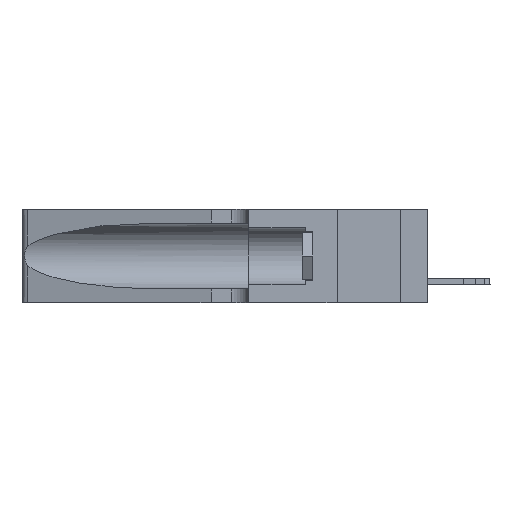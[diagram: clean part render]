
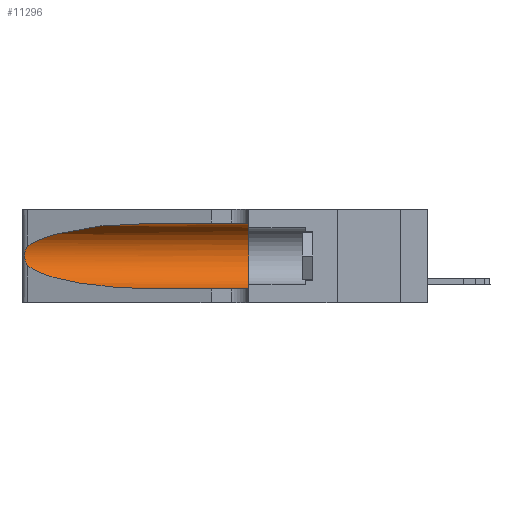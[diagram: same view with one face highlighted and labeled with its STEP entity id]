
A CAD part, left-side view. The second image highlights one B-rep face of the part: STEP entity #11296.
In plain terms, the highlighted cylindrical face has radius 3.308 mm (diameter 6.617 mm), a partial arc.
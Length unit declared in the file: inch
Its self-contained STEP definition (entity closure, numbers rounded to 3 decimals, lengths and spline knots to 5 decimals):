
#935 = CARTESIAN_POINT ( 'NONE',  ( 0.25787, 1.23484, 0.2124 ) ) ;
#1136 = ORIENTED_EDGE ( 'NONE', *, *, #11160, .T. ) ;
#1160 = CARTESIAN_POINT ( 'NONE',  ( 0.25487, 1.22718, 0.14631 ) ) ;
#1245 = VECTOR ( 'NONE', #18800, 39.37008 ) ;
#2476 = CARTESIAN_POINT ( 'NONE',  ( 0.18966, 0.96281, 0.31525 ) ) ;
#2485 = CIRCLE ( 'NONE', #19370, 0.13025 ) ;
#2750 = VERTEX_POINT ( 'NONE', #7155 ) ;
#3383 = CARTESIAN_POINT ( 'NONE',  ( 0.25639, 1.23186, 0.15144 ) ) ;
#3435 = B_SPLINE_CURVE_WITH_KNOTS ( 'NONE', 3,
 ( #26934, #24840, #19873, #935, #5444, #22063, #29535, #5759, #24629, #10415, #15229, #3383, #3483, #20076 ),
 .UNSPECIFIED., .F., .F.,
 ( 4, 2, 2, 2, 2, 2, 4 ),
 ( 0., 0.00027, 0.00053, 0.00107, 0.0016, 0.00187, 0.00214 ),
 .UNSPECIFIED. ) ;
#3483 = CARTESIAN_POINT ( 'NONE',  ( 0.25555, 1.22993, 0.14849 ) ) ;
#3487 = CARTESIAN_POINT ( 'NONE',  ( 0.2373, 1.15595, 0.08982 ) ) ;
#3792 = EDGE_CURVE ( 'NONE', #9569, #2750, #24919, .T. ) ;
#4123 = DIRECTION ( 'NONE',  ( 0., 0., 1. ) ) ;
#4322 = CARTESIAN_POINT ( 'NONE',  ( 0.18966, 0.96281, 0.05475 ) ) ;
#5121 =( BOUNDED_CURVE ( )  B_SPLINE_CURVE ( 3, ( #17701, #3487, #4322, #23492 ),
 .UNSPECIFIED., .F., .T. ) 
 B_SPLINE_CURVE_WITH_KNOTS ( ( 4, 4 ),
 ( 3.44316, 4.71239 ),
 .UNSPECIFIED. ) 
 CURVE ( )  GEOMETRIC_REPRESENTATION_ITEM ( )  RATIONAL_B_SPLINE_CURVE ( ( 1., 0.87, 0.87, 1. ) ) 
 REPRESENTATION_ITEM ( '' )  );
#5444 = CARTESIAN_POINT ( 'NONE',  ( 0.25854, 1.2359, 0.20912 ) ) ;
#5759 = CARTESIAN_POINT ( 'NONE',  ( 0.26075, 1.23896, 0.178 ) ) ;
#6034 = DIRECTION ( 'NONE',  ( 0., 0., -1. ) ) ;
#6055 = EDGE_CURVE ( 'NONE', #29790, #15580, #2485, .T. ) ;
#6140 = ORIENTED_EDGE ( 'NONE', *, *, #18362, .F. ) ;
#7155 = CARTESIAN_POINT ( 'NONE',  ( 0.25487, 1.22718, 0.22369 ) ) ;
#7856 = CYLINDRICAL_SURFACE ( 'NONE', #13748, 0.13025 ) ;
#9201 = DIRECTION ( 'NONE',  ( 0., 1., 0. ) ) ;
#9569 = VERTEX_POINT ( 'NONE', #29063 ) ;
#10415 = CARTESIAN_POINT ( 'NONE',  ( 0.25856, 1.23593, 0.16098 ) ) ;
#11160 = EDGE_CURVE ( 'NONE', #20921, #15580, #15711, .T. ) ;
#11296 = ADVANCED_FACE ( 'NONE', ( #20855 ), #7856, .F. ) ;
#11431 = DIRECTION ( 'NONE',  ( 0., -1., 0. ) ) ;
#11996 = VERTEX_POINT ( 'NONE', #1160 ) ;
#12589 = ORIENTED_EDGE ( 'NONE', *, *, #22698, .T. ) ;
#12838 = EDGE_CURVE ( 'NONE', #11996, #20921, #5121, .T. ) ;
#13206 = CARTESIAN_POINT ( 'NONE',  ( 0.1305, 1.61858, 0.185 ) ) ;
#13689 = CARTESIAN_POINT ( 'NONE',  ( 0.1305, 0.35, 0.185 ) ) ;
#13748 = AXIS2_PLACEMENT_3D ( 'NONE', #13206, #17862, #6034 ) ;
#14402 = CARTESIAN_POINT ( 'NONE',  ( 0.1305, 0.72297, 0.31525 ) ) ;
#14720 = LINE ( 'NONE', #30743, #29181 ) ;
#15229 = CARTESIAN_POINT ( 'NONE',  ( 0.25789, 1.23486, 0.15765 ) ) ;
#15580 = VERTEX_POINT ( 'NONE', #27198 ) ;
#15711 = LINE ( 'NONE', #30462, #1245 ) ;
#16007 = CARTESIAN_POINT ( 'NONE',  ( 0.1305, 0.72297, 0.05475 ) ) ;
#16883 = ORIENTED_EDGE ( 'NONE', *, *, #6055, .F. ) ;
#17701 = CARTESIAN_POINT ( 'NONE',  ( 0.25487, 1.22718, 0.14631 ) ) ;
#17862 = DIRECTION ( 'NONE',  ( 0., -1., 0. ) ) ;
#18316 = EDGE_LOOP ( 'NONE', ( #25067, #12589, #30289, #1136, #16883, #6140 ) ) ;
#18362 = EDGE_CURVE ( 'NONE', #9569, #29790, #14720, .T. ) ;
#18800 = DIRECTION ( 'NONE',  ( 0., -1., 0. ) ) ;
#19036 = CARTESIAN_POINT ( 'NONE',  ( 0.2373, 1.15595, 0.28018 ) ) ;
#19370 = AXIS2_PLACEMENT_3D ( 'NONE', #13689, #9201, #4123 ) ;
#19873 = CARTESIAN_POINT ( 'NONE',  ( 0.25639, 1.23184, 0.21858 ) ) ;
#20076 = CARTESIAN_POINT ( 'NONE',  ( 0.25487, 1.22718, 0.14631 ) ) ;
#20855 = FACE_OUTER_BOUND ( 'NONE', #18316, .T. ) ;
#20921 = VERTEX_POINT ( 'NONE', #16007 ) ;
#22063 = CARTESIAN_POINT ( 'NONE',  ( 0.26018, 1.23835, 0.19895 ) ) ;
#22698 = EDGE_CURVE ( 'NONE', #2750, #11996, #3435, .T. ) ;
#23492 = CARTESIAN_POINT ( 'NONE',  ( 0.1305, 0.72297, 0.05475 ) ) ;
#24629 = CARTESIAN_POINT ( 'NONE',  ( 0.26017, 1.23833, 0.17102 ) ) ;
#24840 = CARTESIAN_POINT ( 'NONE',  ( 0.25555, 1.22994, 0.2215 ) ) ;
#24919 =( BOUNDED_CURVE ( )  B_SPLINE_CURVE ( 3, ( #14402, #2476, #19036, #26406 ),
 .UNSPECIFIED., .F., .T. ) 
 B_SPLINE_CURVE_WITH_KNOTS ( ( 4, 4 ),
 ( 1.5708, 2.84003 ),
 .UNSPECIFIED. ) 
 CURVE ( )  GEOMETRIC_REPRESENTATION_ITEM ( )  RATIONAL_B_SPLINE_CURVE ( ( 1., 0.87, 0.87, 1. ) ) 
 REPRESENTATION_ITEM ( '' )  );
#25067 = ORIENTED_EDGE ( 'NONE', *, *, #3792, .T. ) ;
#26406 = CARTESIAN_POINT ( 'NONE',  ( 0.25487, 1.22718, 0.22369 ) ) ;
#26934 = CARTESIAN_POINT ( 'NONE',  ( 0.25487, 1.22718, 0.22369 ) ) ;
#27198 = CARTESIAN_POINT ( 'NONE',  ( 0.1305, 0.35, 0.05475 ) ) ;
#27576 = CARTESIAN_POINT ( 'NONE',  ( 0.1305, 0.35, 0.31525 ) ) ;
#29063 = CARTESIAN_POINT ( 'NONE',  ( 0.1305, 0.72297, 0.31525 ) ) ;
#29181 = VECTOR ( 'NONE', #11431, 39.37008 ) ;
#29535 = CARTESIAN_POINT ( 'NONE',  ( 0.26075, 1.23896, 0.19203 ) ) ;
#29790 = VERTEX_POINT ( 'NONE', #27576 ) ;
#30289 = ORIENTED_EDGE ( 'NONE', *, *, #12838, .T. ) ;
#30462 = CARTESIAN_POINT ( 'NONE',  ( 0.1305, 1.61858, 0.05475 ) ) ;
#30743 = CARTESIAN_POINT ( 'NONE',  ( 0.1305, 1.61858, 0.31525 ) ) ;
